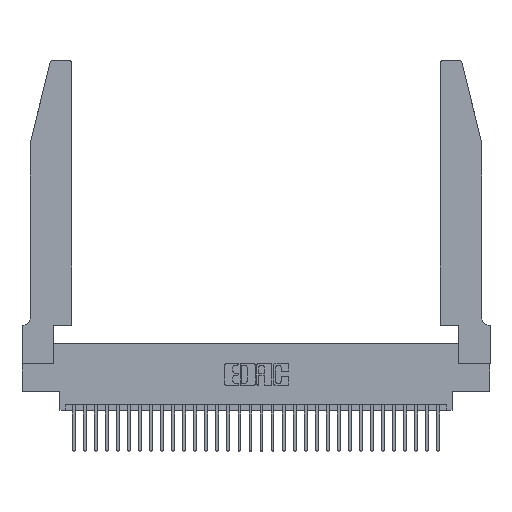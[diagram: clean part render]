
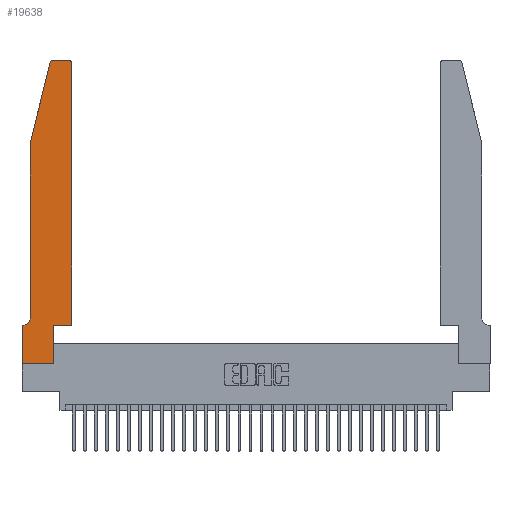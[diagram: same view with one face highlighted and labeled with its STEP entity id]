
A CAD part, top view. The second image highlights one B-rep face of the part: STEP entity #19638.
In plain terms, the highlighted planar face has unit normal (0, 0, 1).
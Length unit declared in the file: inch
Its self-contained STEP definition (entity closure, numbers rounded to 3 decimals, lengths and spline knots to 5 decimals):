
#921 = CARTESIAN_POINT ( 'NONE',  ( 0.284, 2.75, 0.37 ) ) ;
#1257 = CARTESIAN_POINT ( 'NONE',  ( 0.4505, 0.35, 0.37 ) ) ;
#1478 = CARTESIAN_POINT ( 'NONE',  ( 0.2605, 2.75, 0.37 ) ) ;
#1545 = EDGE_CURVE ( 'NONE', #8308, #22562, #28841, .T. ) ;
#1764 = EDGE_CURVE ( 'NONE', #8389, #16477, #12241, .T. ) ;
#1954 = VECTOR ( 'NONE', #27413, 39.37008 ) ;
#3423 = CARTESIAN_POINT ( 'NONE',  ( 0.0755, 2., 0.37 ) ) ;
#4388 = VERTEX_POINT ( 'NONE', #20144 ) ;
#4647 = DIRECTION ( 'NONE',  ( 1., 0., 0. ) ) ;
#4899 = EDGE_LOOP ( 'NONE', ( #12609, #32604, #29377, #20826, #15471, #18425, #7425, #15302, #18225, #19316, #14177, #11194 ) ) ;
#5167 = VECTOR ( 'NONE', #22642, 39.37008 ) ;
#5312 = DIRECTION ( 'NONE',  ( 0., 0., 1. ) ) ;
#5501 = EDGE_CURVE ( 'NONE', #21975, #31168, #20467, .T. ) ;
#5590 = CARTESIAN_POINT ( 'NONE',  ( 0., 0.35, 0.37 ) ) ;
#5595 = EDGE_CURVE ( 'NONE', #22562, #26502, #26018, .T. ) ;
#5844 = EDGE_CURVE ( 'NONE', #4388, #15192, #16909, .T. ) ;
#5902 = CARTESIAN_POINT ( 'NONE',  ( 0.4205, 2.75, 0.37 ) ) ;
#6544 = AXIS2_PLACEMENT_3D ( 'NONE', #28094, #7716, #10414 ) ;
#7079 = CARTESIAN_POINT ( 'NONE',  ( 0.284, 2.72, 0.37 ) ) ;
#7267 = EDGE_CURVE ( 'NONE', #16477, #4388, #8132, .T. ) ;
#7425 = ORIENTED_EDGE ( 'NONE', *, *, #5844, .T. ) ;
#7716 = DIRECTION ( 'NONE',  ( 0., 0., -1. ) ) ;
#8132 = LINE ( 'NONE', #31497, #13279 ) ;
#8308 = VERTEX_POINT ( 'NONE', #921 ) ;
#8389 = VERTEX_POINT ( 'NONE', #32330 ) ;
#8582 = CARTESIAN_POINT ( 'NONE',  ( 0., 0., 0.37 ) ) ;
#9474 = AXIS2_PLACEMENT_3D ( 'NONE', #5590, #5312, #23047 ) ;
#10085 = EDGE_CURVE ( 'NONE', #17556, #8308, #14708, .T. ) ;
#10156 = VERTEX_POINT ( 'NONE', #24192 ) ;
#10414 = DIRECTION ( 'NONE',  ( -1., 0., 0. ) ) ;
#11160 = CARTESIAN_POINT ( 'NONE',  ( 0., 0., 0.37 ) ) ;
#11169 = DIRECTION ( 'NONE',  ( 1., 0., 0. ) ) ;
#11194 = ORIENTED_EDGE ( 'NONE', *, *, #26874, .T. ) ;
#11396 = DIRECTION ( 'NONE',  ( 0., -1., 0. ) ) ;
#12058 = CARTESIAN_POINT ( 'NONE',  ( 0.0055, 0.35, 0.37 ) ) ;
#12221 = DIRECTION ( 'NONE',  ( 0., 0., 1. ) ) ;
#12241 = CIRCLE ( 'NONE', #6544, 0.07 ) ;
#12319 = VECTOR ( 'NONE', #26506, 39.37008 ) ;
#12410 = CIRCLE ( 'NONE', #32433, 0.03 ) ;
#12609 = ORIENTED_EDGE ( 'NONE', *, *, #10085, .T. ) ;
#12829 = DIRECTION ( 'NONE',  ( 0., 1., 0. ) ) ;
#13279 = VECTOR ( 'NONE', #31275, 39.37008 ) ;
#13591 = FACE_OUTER_BOUND ( 'NONE', #4899, .T. ) ;
#14177 = ORIENTED_EDGE ( 'NONE', *, *, #23136, .T. ) ;
#14708 = LINE ( 'NONE', #1478, #12319 ) ;
#14710 = VECTOR ( 'NONE', #12829, 39.37008 ) ;
#15192 = VERTEX_POINT ( 'NONE', #8582 ) ;
#15302 = ORIENTED_EDGE ( 'NONE', *, *, #23651, .T. ) ;
#15471 = ORIENTED_EDGE ( 'NONE', *, *, #1764, .T. ) ;
#16477 = VERTEX_POINT ( 'NONE', #12058 ) ;
#16909 = LINE ( 'NONE', #11160, #29558 ) ;
#17556 = VERTEX_POINT ( 'NONE', #5902 ) ;
#18100 = DIRECTION ( 'NONE',  ( 1., 0., 0. ) ) ;
#18225 = ORIENTED_EDGE ( 'NONE', *, *, #28948, .T. ) ;
#18425 = ORIENTED_EDGE ( 'NONE', *, *, #7267, .T. ) ;
#19316 = ORIENTED_EDGE ( 'NONE', *, *, #5501, .T. ) ;
#19638 = ADVANCED_FACE ( 'NONE', ( #13591 ), #32585, .T. ) ;
#20144 = CARTESIAN_POINT ( 'NONE',  ( 0., 0.35, 0.37 ) ) ;
#20301 = CARTESIAN_POINT ( 'NONE',  ( 0.25487, 2.72718, 0.37 ) ) ;
#20467 = LINE ( 'NONE', #1257, #21282 ) ;
#20596 = LINE ( 'NONE', #30616, #14710 ) ;
#20826 = ORIENTED_EDGE ( 'NONE', *, *, #29249, .T. ) ;
#21282 = VECTOR ( 'NONE', #11169, 39.37008 ) ;
#21455 = CARTESIAN_POINT ( 'NONE',  ( 0.0755, 2., 0.37 ) ) ;
#21888 = CARTESIAN_POINT ( 'NONE',  ( 0.4505, 0.35, 0.37 ) ) ;
#21975 = VERTEX_POINT ( 'NONE', #32428 ) ;
#22562 = VERTEX_POINT ( 'NONE', #20301 ) ;
#22642 = DIRECTION ( 'NONE',  ( 0., 1., 0. ) ) ;
#22766 = AXIS2_PLACEMENT_3D ( 'NONE', #7079, #12221, #18100 ) ;
#23047 = DIRECTION ( 'NONE',  ( 1., 0., 0. ) ) ;
#23136 = EDGE_CURVE ( 'NONE', #31168, #10156, #27663, .T. ) ;
#23651 = EDGE_CURVE ( 'NONE', #15192, #27315, #30388, .T. ) ;
#23775 = CARTESIAN_POINT ( 'NONE',  ( 0.0755, 2., 0.37 ) ) ;
#24192 = CARTESIAN_POINT ( 'NONE',  ( 0.4505, 2.72, 0.37 ) ) ;
#25336 = VECTOR ( 'NONE', #31374, 39.37008 ) ;
#26018 = LINE ( 'NONE', #23775, #1954 ) ;
#26502 = VERTEX_POINT ( 'NONE', #3423 ) ;
#26506 = DIRECTION ( 'NONE',  ( -1., 0., 0. ) ) ;
#26874 = EDGE_CURVE ( 'NONE', #10156, #17556, #12410, .T. ) ;
#27208 = CARTESIAN_POINT ( 'NONE',  ( 0.2865, 0., 0.37 ) ) ;
#27313 = LINE ( 'NONE', #21455, #25336 ) ;
#27315 = VERTEX_POINT ( 'NONE', #27208 ) ;
#27413 = DIRECTION ( 'NONE',  ( -0.239, -0.971, 0. ) ) ;
#27663 = LINE ( 'NONE', #32253, #5167 ) ;
#28094 = CARTESIAN_POINT ( 'NONE',  ( 0.0055, 0.42, 0.37 ) ) ;
#28841 = CIRCLE ( 'NONE', #22766, 0.03 ) ;
#28948 = EDGE_CURVE ( 'NONE', #27315, #21975, #20596, .T. ) ;
#29249 = EDGE_CURVE ( 'NONE', #26502, #8389, #27313, .T. ) ;
#29365 = CARTESIAN_POINT ( 'NONE',  ( 0., 0., 0.37 ) ) ;
#29377 = ORIENTED_EDGE ( 'NONE', *, *, #5595, .T. ) ;
#29558 = VECTOR ( 'NONE', #11396, 39.37008 ) ;
#29898 = DIRECTION ( 'NONE',  ( 0., 0., 1. ) ) ;
#30388 = LINE ( 'NONE', #29365, #31974 ) ;
#30616 = CARTESIAN_POINT ( 'NONE',  ( 0.2865, 0.35, 0.37 ) ) ;
#31168 = VERTEX_POINT ( 'NONE', #21888 ) ;
#31275 = DIRECTION ( 'NONE',  ( -1., 0., 0. ) ) ;
#31374 = DIRECTION ( 'NONE',  ( 0., -1., 0. ) ) ;
#31451 = DIRECTION ( 'NONE',  ( 1., 0., 0. ) ) ;
#31497 = CARTESIAN_POINT ( 'NONE',  ( 0.0755, 0.35, 0.37 ) ) ;
#31974 = VECTOR ( 'NONE', #31451, 39.37008 ) ;
#32253 = CARTESIAN_POINT ( 'NONE',  ( 0.4505, 0.35, 0.37 ) ) ;
#32306 = CARTESIAN_POINT ( 'NONE',  ( 0.4205, 2.72, 0.37 ) ) ;
#32330 = CARTESIAN_POINT ( 'NONE',  ( 0.0755, 0.42, 0.37 ) ) ;
#32428 = CARTESIAN_POINT ( 'NONE',  ( 0.2865, 0.35, 0.37 ) ) ;
#32433 = AXIS2_PLACEMENT_3D ( 'NONE', #32306, #29898, #4647 ) ;
#32585 = PLANE ( 'NONE',  #9474 ) ;
#32604 = ORIENTED_EDGE ( 'NONE', *, *, #1545, .T. ) ;
